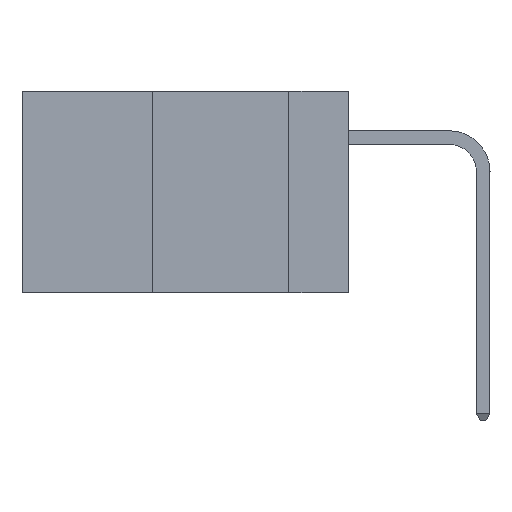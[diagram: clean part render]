
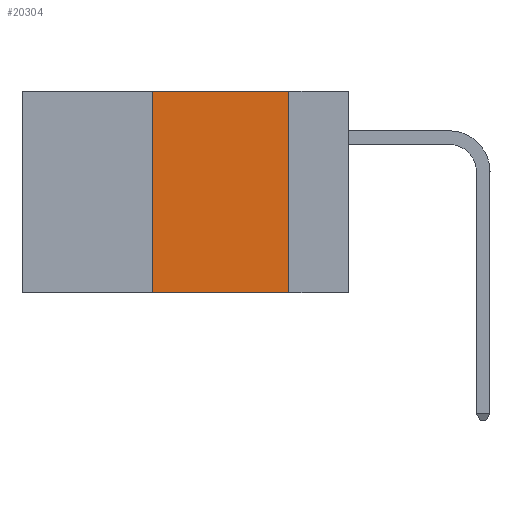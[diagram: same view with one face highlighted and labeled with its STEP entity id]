
A CAD part, left-side view. The second image highlights one B-rep face of the part: STEP entity #20304.
In plain terms, the highlighted planar face has unit normal (-1, 0, 0).
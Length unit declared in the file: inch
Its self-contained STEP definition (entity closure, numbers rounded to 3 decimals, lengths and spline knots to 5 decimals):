
#416 = VERTEX_POINT ( 'NONE', #19255 ) ;
#2122 = VECTOR ( 'NONE', #10683, 39.37008 ) ;
#2380 = EDGE_LOOP ( 'NONE', ( #15780, #3164, #12985, #14009 ) ) ;
#2390 = LINE ( 'NONE', #27556, #14338 ) ;
#2516 = VECTOR ( 'NONE', #26876, 39.37008 ) ;
#2852 = LINE ( 'NONE', #8439, #2122 ) ;
#3164 = ORIENTED_EDGE ( 'NONE', *, *, #6575, .F. ) ;
#3454 = LINE ( 'NONE', #4205, #8766 ) ;
#3835 = CARTESIAN_POINT ( 'NONE',  ( 0., 0.11, 0. ) ) ;
#4205 = CARTESIAN_POINT ( 'NONE',  ( 0., 0.6, -0.37 ) ) ;
#5157 = VERTEX_POINT ( 'NONE', #5457 ) ;
#5457 = CARTESIAN_POINT ( 'NONE',  ( 0., 0.36, 0. ) ) ;
#6575 = EDGE_CURVE ( 'NONE', #5157, #16615, #20984, .T. ) ;
#6918 = CARTESIAN_POINT ( 'NONE',  ( 0., 0.11, -0.37 ) ) ;
#6996 = CARTESIAN_POINT ( 'NONE',  ( 0., 0.6, 0. ) ) ;
#7811 = VERTEX_POINT ( 'NONE', #6918 ) ;
#8439 = CARTESIAN_POINT ( 'NONE',  ( 0., 0.11, 0. ) ) ;
#8766 = VECTOR ( 'NONE', #13103, 39.37008 ) ;
#9335 = FACE_OUTER_BOUND ( 'NONE', #2380, .T. ) ;
#10683 = DIRECTION ( 'NONE',  ( 0., 0., -1. ) ) ;
#11116 = PLANE ( 'NONE',  #20213 ) ;
#12985 = ORIENTED_EDGE ( 'NONE', *, *, #18735, .F. ) ;
#13103 = DIRECTION ( 'NONE',  ( 0., -1., 0. ) ) ;
#13325 = CARTESIAN_POINT ( 'NONE',  ( 0., 0.6, 0. ) ) ;
#14009 = ORIENTED_EDGE ( 'NONE', *, *, #24565, .T. ) ;
#14338 = VECTOR ( 'NONE', #14470, 39.37008 ) ;
#14470 = DIRECTION ( 'NONE',  ( 0., 0., 1. ) ) ;
#15552 = DIRECTION ( 'NONE',  ( 0., 0., -1. ) ) ;
#15780 = ORIENTED_EDGE ( 'NONE', *, *, #17267, .F. ) ;
#16615 = VERTEX_POINT ( 'NONE', #3835 ) ;
#17267 = EDGE_CURVE ( 'NONE', #16615, #7811, #2852, .T. ) ;
#18735 = EDGE_CURVE ( 'NONE', #416, #5157, #2390, .T. ) ;
#19255 = CARTESIAN_POINT ( 'NONE',  ( 0., 0.36, -0.37 ) ) ;
#20213 = AXIS2_PLACEMENT_3D ( 'NONE', #13325, #28606, #15552 ) ;
#20304 = ADVANCED_FACE ( 'NONE', ( #9335 ), #11116, .F. ) ;
#20984 = LINE ( 'NONE', #6996, #2516 ) ;
#24565 = EDGE_CURVE ( 'NONE', #416, #7811, #3454, .T. ) ;
#26876 = DIRECTION ( 'NONE',  ( 0., -1., 0. ) ) ;
#27556 = CARTESIAN_POINT ( 'NONE',  ( 0., 0.36, 0. ) ) ;
#28606 = DIRECTION ( 'NONE',  ( 1., 0., 0. ) ) ;
